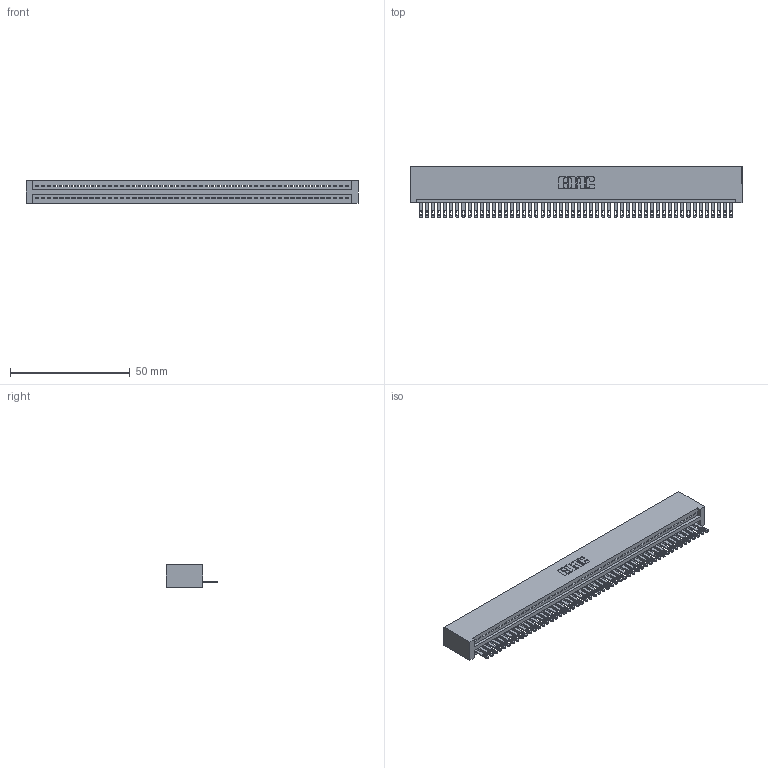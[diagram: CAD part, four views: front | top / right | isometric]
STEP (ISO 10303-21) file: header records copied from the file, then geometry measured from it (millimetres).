
FILE_DESCRIPTION (( 'STEP AP203' ), '1' );
FILE_NAME ('345-052-500-101.STEP', '2019-10-09T17:01:09', ( '' ), ( '' ), 'SwSTEP 2.0', 'SolidWorks 2016', '' );
FILE_SCHEMA (( 'CONFIG_CONTROL_DESIGN' ));
Length unit declared in the file: inch
Products named in the file (3): 345-292-001_345-293-100; 345 Part_No Mounting Lugs; 345-052-500-101
Assembly tree (53 placements, depth 2):
  345-052-500-101
    345 Part_No Mounting Lugs
    345-292-001_345-293-100  x52
Bounding box: 138.68 x 21.51 x 9.4 mm (x, y, z)
Volume: 13870.8 mm3; surface area: 18875.9 mm2
Topology: 53 solids, 53 shells, 2926 faces, 9053 edges, 6034 vertices
Faces by surface type: plane 1844, cylinder 1082
Entity records: 37443 total; most frequent: CARTESIAN_POINT 6492, ORIENTED_EDGE 6478, DIRECTION 5651, EDGE_CURVE 3239, LINE 2903, VECTOR 2903, VERTEX_POINT 2158, AXIS2_PLACEMENT_3D 1374
